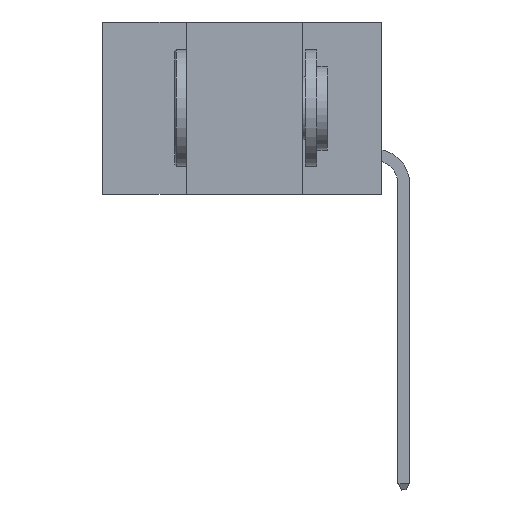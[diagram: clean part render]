
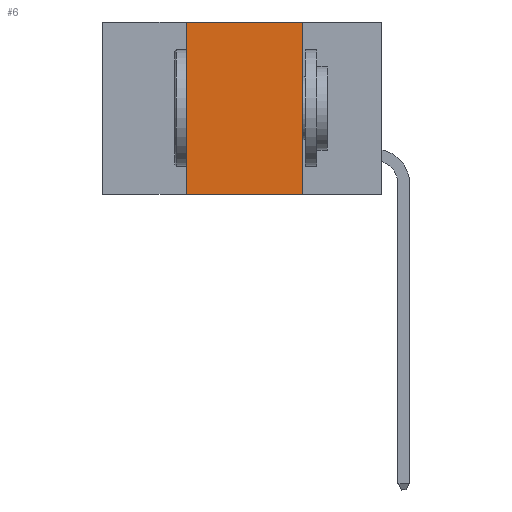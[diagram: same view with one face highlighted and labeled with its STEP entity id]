
A CAD part, left-side view. The second image highlights one B-rep face of the part: STEP entity #6.
In plain terms, the highlighted planar face has unit normal (-1, 0, 0).
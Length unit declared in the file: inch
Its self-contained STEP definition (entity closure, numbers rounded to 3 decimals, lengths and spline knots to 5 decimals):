
#6 = ADVANCED_FACE ( 'NONE', ( #7045 ), #4983, .F. ) ;
#124 = ORIENTED_EDGE ( 'NONE', *, *, #3999, .F. ) ;
#981 = EDGE_LOOP ( 'NONE', ( #124, #3242, #7645, #3609 ) ) ;
#1056 = VECTOR ( 'NONE', #12618, 39.37008 ) ;
#1590 = CARTESIAN_POINT ( 'NONE',  ( 0., 0.17, 0. ) ) ;
#1672 = DIRECTION ( 'NONE',  ( 0., 0., -1. ) ) ;
#1921 = DIRECTION ( 'NONE',  ( 0., -1., 0. ) ) ;
#2705 = CARTESIAN_POINT ( 'NONE',  ( 0., 0.17, 0. ) ) ;
#3242 = ORIENTED_EDGE ( 'NONE', *, *, #13042, .F. ) ;
#3312 = CARTESIAN_POINT ( 'NONE',  ( 0., 0.17, -0.37 ) ) ;
#3609 = ORIENTED_EDGE ( 'NONE', *, *, #4868, .T. ) ;
#3999 = EDGE_CURVE ( 'NONE', #14035, #12377, #6584, .T. ) ;
#4825 = VECTOR ( 'NONE', #1921, 39.37008 ) ;
#4868 = EDGE_CURVE ( 'NONE', #5780, #12377, #10952, .T. ) ;
#4983 = PLANE ( 'NONE',  #5535 ) ;
#5535 = AXIS2_PLACEMENT_3D ( 'NONE', #8350, #12914, #7385 ) ;
#5780 = VERTEX_POINT ( 'NONE', #7393 ) ;
#6439 = VECTOR ( 'NONE', #12574, 39.37008 ) ;
#6584 = LINE ( 'NONE', #2705, #11822 ) ;
#7045 = FACE_OUTER_BOUND ( 'NONE', #981, .T. ) ;
#7385 = DIRECTION ( 'NONE',  ( 0., 0., -1. ) ) ;
#7393 = CARTESIAN_POINT ( 'NONE',  ( 0., 0.42, -0.37 ) ) ;
#7545 = CARTESIAN_POINT ( 'NONE',  ( 0., 0.6, -0.37 ) ) ;
#7645 = ORIENTED_EDGE ( 'NONE', *, *, #10792, .F. ) ;
#8131 = VERTEX_POINT ( 'NONE', #10660 ) ;
#8189 = LINE ( 'NONE', #10229, #6439 ) ;
#8350 = CARTESIAN_POINT ( 'NONE',  ( 0., 0.6, 0. ) ) ;
#10229 = CARTESIAN_POINT ( 'NONE',  ( 0., 0.6, 0. ) ) ;
#10660 = CARTESIAN_POINT ( 'NONE',  ( 0., 0.42, 0. ) ) ;
#10792 = EDGE_CURVE ( 'NONE', #5780, #8131, #11449, .T. ) ;
#10952 = LINE ( 'NONE', #7545, #4825 ) ;
#11162 = CARTESIAN_POINT ( 'NONE',  ( 0., 0.42, 0. ) ) ;
#11449 = LINE ( 'NONE', #11162, #1056 ) ;
#11822 = VECTOR ( 'NONE', #1672, 39.37008 ) ;
#12377 = VERTEX_POINT ( 'NONE', #3312 ) ;
#12574 = DIRECTION ( 'NONE',  ( 0., -1., 0. ) ) ;
#12618 = DIRECTION ( 'NONE',  ( 0., 0., 1. ) ) ;
#12914 = DIRECTION ( 'NONE',  ( 1., 0., 0. ) ) ;
#13042 = EDGE_CURVE ( 'NONE', #8131, #14035, #8189, .T. ) ;
#14035 = VERTEX_POINT ( 'NONE', #1590 ) ;
